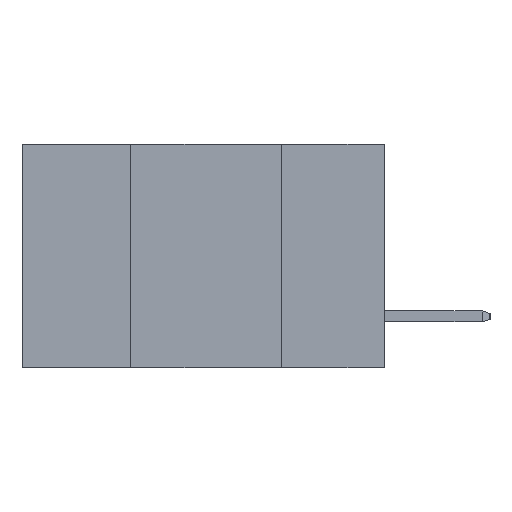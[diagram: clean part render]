
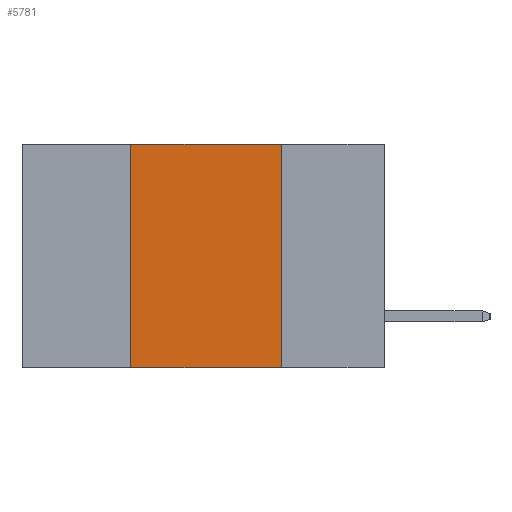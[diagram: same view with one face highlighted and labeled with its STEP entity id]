
A CAD part, left-side view. The second image highlights one B-rep face of the part: STEP entity #5781.
In plain terms, the highlighted planar face has unit normal (-1, 0, 0).
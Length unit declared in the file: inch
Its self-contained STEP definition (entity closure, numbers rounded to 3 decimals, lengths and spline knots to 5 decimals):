
#873 = LINE ( 'NONE', #4801, #8667 ) ;
#2047 = VERTEX_POINT ( 'NONE', #15012 ) ;
#3726 = EDGE_CURVE ( 'NONE', #14117, #2047, #18174, .T. ) ;
#4801 = CARTESIAN_POINT ( 'NONE',  ( 0., 0.17, -0.37 ) ) ;
#4817 = VERTEX_POINT ( 'NONE', #16764 ) ;
#5197 = VERTEX_POINT ( 'NONE', #13087 ) ;
#5661 = CARTESIAN_POINT ( 'NONE',  ( 0., 0.6, 0. ) ) ;
#5757 = EDGE_CURVE ( 'NONE', #14117, #4817, #8125, .T. ) ;
#5781 = ADVANCED_FACE ( 'NONE', ( #19245 ), #8171, .F. ) ;
#7143 = AXIS2_PLACEMENT_3D ( 'NONE', #8323, #8168, #8149 ) ;
#7490 = ORIENTED_EDGE ( 'NONE', *, *, #11929, .F. ) ;
#8125 = LINE ( 'NONE', #8461, #16281 ) ;
#8149 = DIRECTION ( 'NONE',  ( 0., 0., -1. ) ) ;
#8168 = DIRECTION ( 'NONE',  ( 1., 0., 0. ) ) ;
#8171 = PLANE ( 'NONE',  #7143 ) ;
#8323 = CARTESIAN_POINT ( 'NONE',  ( 0., 0.6, 0. ) ) ;
#8329 = DIRECTION ( 'NONE',  ( 0., 0., 1. ) ) ;
#8461 = CARTESIAN_POINT ( 'NONE',  ( 0., 0.42, -0.37 ) ) ;
#8485 = LINE ( 'NONE', #5661, #12567 ) ;
#8667 = VECTOR ( 'NONE', #18465, 39.37008 ) ;
#8938 = ORIENTED_EDGE ( 'NONE', *, *, #5757, .F. ) ;
#9639 = VECTOR ( 'NONE', #18894, 39.37008 ) ;
#11929 = EDGE_CURVE ( 'NONE', #4817, #5197, #8485, .T. ) ;
#12567 = VECTOR ( 'NONE', #14869, 39.37008 ) ;
#13087 = CARTESIAN_POINT ( 'NONE',  ( 0., 0.17, 0. ) ) ;
#13837 = EDGE_LOOP ( 'NONE', ( #14230, #7490, #8938, #17976 ) ) ;
#14117 = VERTEX_POINT ( 'NONE', #16192 ) ;
#14230 = ORIENTED_EDGE ( 'NONE', *, *, #16041, .F. ) ;
#14869 = DIRECTION ( 'NONE',  ( 0., -1., 0. ) ) ;
#15012 = CARTESIAN_POINT ( 'NONE',  ( 0., 0.17, -0.37 ) ) ;
#16041 = EDGE_CURVE ( 'NONE', #5197, #2047, #873, .T. ) ;
#16192 = CARTESIAN_POINT ( 'NONE',  ( 0., 0.42, -0.37 ) ) ;
#16281 = VECTOR ( 'NONE', #8329, 39.37008 ) ;
#16764 = CARTESIAN_POINT ( 'NONE',  ( 0., 0.42, 0. ) ) ;
#17976 = ORIENTED_EDGE ( 'NONE', *, *, #3726, .T. ) ;
#18174 = LINE ( 'NONE', #19790, #9639 ) ;
#18465 = DIRECTION ( 'NONE',  ( 0., 0., -1. ) ) ;
#18894 = DIRECTION ( 'NONE',  ( 0., -1., 0. ) ) ;
#19245 = FACE_OUTER_BOUND ( 'NONE', #13837, .T. ) ;
#19790 = CARTESIAN_POINT ( 'NONE',  ( 0., 0.6, -0.37 ) ) ;
